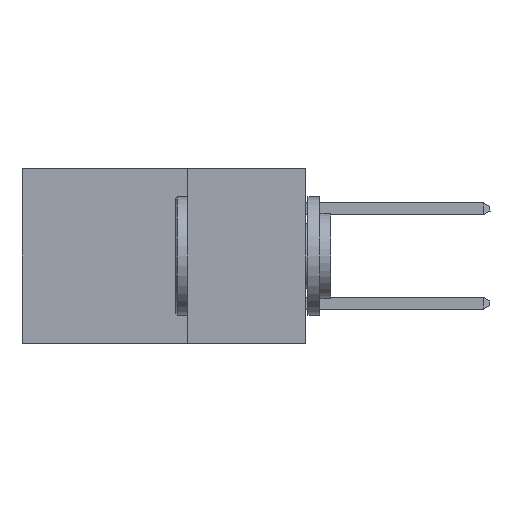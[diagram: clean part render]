
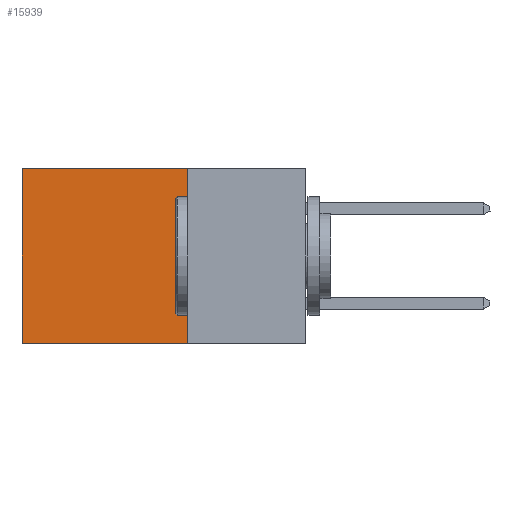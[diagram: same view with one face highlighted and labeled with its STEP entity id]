
A CAD part, left-side view. The second image highlights one B-rep face of the part: STEP entity #15939.
In plain terms, the highlighted planar face has unit normal (-1, 0, 0).
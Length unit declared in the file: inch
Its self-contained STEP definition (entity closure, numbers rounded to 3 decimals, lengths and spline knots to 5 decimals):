
#125 = VECTOR ( 'NONE', #17166, 39.37008 ) ;
#805 = VERTEX_POINT ( 'NONE', #5618 ) ;
#3015 = ORIENTED_EDGE ( 'NONE', *, *, #15565, .F. ) ;
#3885 = CARTESIAN_POINT ( 'NONE',  ( 0.298, 0.25, -0.37 ) ) ;
#4535 = VERTEX_POINT ( 'NONE', #11657 ) ;
#4891 = DIRECTION ( 'NONE',  ( 1., 0., 0. ) ) ;
#5095 = EDGE_CURVE ( 'NONE', #15687, #4535, #10163, .T. ) ;
#5618 = CARTESIAN_POINT ( 'NONE',  ( 0.298, 0.6, 0. ) ) ;
#6529 = ORIENTED_EDGE ( 'NONE', *, *, #5095, .F. ) ;
#6712 = DIRECTION ( 'NONE',  ( 0., 0., -1. ) ) ;
#8074 = CARTESIAN_POINT ( 'NONE',  ( 0.298, 0.25, 0. ) ) ;
#8703 = ORIENTED_EDGE ( 'NONE', *, *, #11808, .T. ) ;
#9184 = PLANE ( 'NONE',  #22690 ) ;
#10163 = LINE ( 'NONE', #21020, #26824 ) ;
#10688 = CARTESIAN_POINT ( 'NONE',  ( 0.298, 0.25, 0. ) ) ;
#11136 = CARTESIAN_POINT ( 'NONE',  ( 0.298, 0.6, -0.37 ) ) ;
#11657 = CARTESIAN_POINT ( 'NONE',  ( 0.298, 0.25, -0.37 ) ) ;
#11808 = EDGE_CURVE ( 'NONE', #15687, #805, #18969, .T. ) ;
#12104 = DIRECTION ( 'NONE',  ( 0., 0., -1. ) ) ;
#13011 = CARTESIAN_POINT ( 'NONE',  ( 0.298, 0.6, 0. ) ) ;
#13915 = CARTESIAN_POINT ( 'NONE',  ( 0.298, 0.25, 0. ) ) ;
#13992 = ORIENTED_EDGE ( 'NONE', *, *, #18299, .T. ) ;
#14015 = EDGE_LOOP ( 'NONE', ( #13992, #3015, #6529, #8703 ) ) ;
#15565 = EDGE_CURVE ( 'NONE', #4535, #21905, #19099, .T. ) ;
#15687 = VERTEX_POINT ( 'NONE', #10688 ) ;
#15939 = ADVANCED_FACE ( 'NONE', ( #21214 ), #9184, .F. ) ;
#17166 = DIRECTION ( 'NONE',  ( 0., 1., 0. ) ) ;
#18299 = EDGE_CURVE ( 'NONE', #805, #21905, #27337, .T. ) ;
#18969 = LINE ( 'NONE', #8074, #125 ) ;
#19099 = LINE ( 'NONE', #3885, #23674 ) ;
#21020 = CARTESIAN_POINT ( 'NONE',  ( 0.298, 0.25, 0. ) ) ;
#21214 = FACE_OUTER_BOUND ( 'NONE', #14015, .T. ) ;
#21347 = VECTOR ( 'NONE', #22213, 39.37008 ) ;
#21905 = VERTEX_POINT ( 'NONE', #11136 ) ;
#22213 = DIRECTION ( 'NONE',  ( 0., 0., -1. ) ) ;
#22690 = AXIS2_PLACEMENT_3D ( 'NONE', #13915, #4891, #6712 ) ;
#23674 = VECTOR ( 'NONE', #24420, 39.37008 ) ;
#24420 = DIRECTION ( 'NONE',  ( 0., 1., 0. ) ) ;
#26824 = VECTOR ( 'NONE', #12104, 39.37008 ) ;
#27337 = LINE ( 'NONE', #13011, #21347 ) ;
